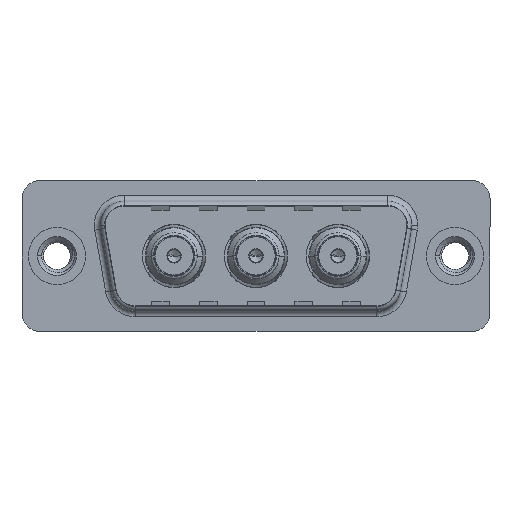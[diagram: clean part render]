
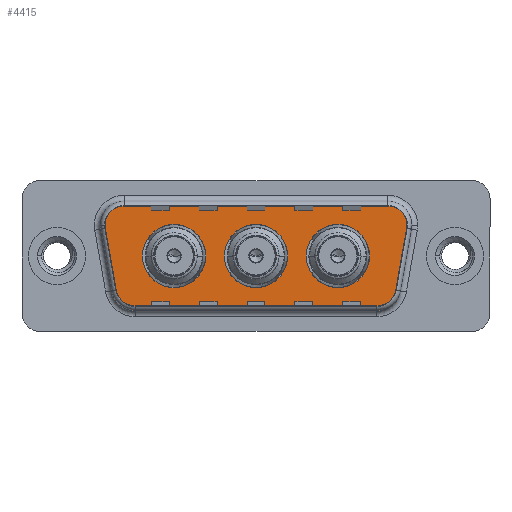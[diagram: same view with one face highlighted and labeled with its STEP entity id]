
A CAD part, top view. The second image highlights one B-rep face of the part: STEP entity #4415.
In plain terms, the highlighted planar face has unit normal (0, 0, 1).
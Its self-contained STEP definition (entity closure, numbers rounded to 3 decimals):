
#24 = ORIENTED_EDGE ( 'NONE', *, *, #8987, .F. ) ;
#173 = DIRECTION ( 'NONE',  ( 0., 0., 1. ) ) ;
#301 = DIRECTION ( 'NONE',  ( 0., 0., 1. ) ) ;
#363 = CIRCLE ( 'NONE', #13225, 2.65 ) ;
#427 = CARTESIAN_POINT ( 'NONE',  ( 16.65, 0., 0. ) ) ;
#432 = ORIENTED_EDGE ( 'NONE', *, *, #10453, .F. ) ;
#610 = AXIS2_PLACEMENT_3D ( 'NONE', #3767, #6325, #14634 ) ;
#1162 = DIRECTION ( 'NONE',  ( 0., 0., 1. ) ) ;
#1231 = AXIS2_PLACEMENT_3D ( 'NONE', #14390, #301, #10093 ) ;
#1262 = VERTEX_POINT ( 'NONE', #11161 ) ;
#1274 = CARTESIAN_POINT ( 'NONE',  ( 16.65, 0., 0. ) ) ;
#1303 = CARTESIAN_POINT ( 'NONE',  ( 7.15, 0., 0. ) ) ;
#1335 = DIRECTION ( 'NONE',  ( 0., 0., 1. ) ) ;
#1395 = CIRCLE ( 'NONE', #10770, 2.65 ) ;
#1501 = VECTOR ( 'NONE', #5473, 1000. ) ;
#1601 = CIRCLE ( 'NONE', #610, 2. ) ;
#1887 = AXIS2_PLACEMENT_3D ( 'NONE', #13021, #1162, #8384 ) ;
#1901 = CARTESIAN_POINT ( 'NONE',  ( 23.5, 0., 0. ) ) ;
#1971 = VERTEX_POINT ( 'NONE', #10240 ) ;
#1978 = ORIENTED_EDGE ( 'NONE', *, *, #2971, .F. ) ;
#2191 = CARTESIAN_POINT ( 'NONE',  ( 27.889, 2.9, 0. ) ) ;
#2239 = LINE ( 'NONE', #8644, #8415 ) ;
#2399 = FACE_BOUND ( 'NONE', #2434, .T. ) ;
#2434 = EDGE_LOOP ( 'NONE', ( #14392, #24 ) ) ;
#2557 = VERTEX_POINT ( 'NONE', #5701 ) ;
#2687 = EDGE_LOOP ( 'NONE', ( #15388, #13432, #11406, #6862, #10670, #14062, #4432, #4471, #3535 ) ) ;
#2800 = DIRECTION ( 'NONE',  ( 0., 0., 1. ) ) ;
#2971 = EDGE_CURVE ( 'NONE', #1262, #7063, #11347, .T. ) ;
#2984 = VERTEX_POINT ( 'NONE', #13394 ) ;
#3138 = DIRECTION ( 'NONE',  ( 1., 0., 0. ) ) ;
#3183 = CIRCLE ( 'NONE', #15477, 2. ) ;
#3528 = VECTOR ( 'NONE', #8202, 1000. ) ;
#3535 = ORIENTED_EDGE ( 'NONE', *, *, #8207, .T. ) ;
#3587 = CIRCLE ( 'NONE', #4645, 2.65 ) ;
#3723 = DIRECTION ( 'NONE',  ( 0.174, 0.985, 0. ) ) ;
#3767 = CARTESIAN_POINT ( 'NONE',  ( 5.411, 2.9, 0. ) ) ;
#3775 = CIRCLE ( 'NONE', #5178, 2.65 ) ;
#3802 = EDGE_CURVE ( 'NONE', #4691, #5275, #3183, .T. ) ;
#3902 = DIRECTION ( 'NONE',  ( 0., 0., 1. ) ) ;
#3920 = LINE ( 'NONE', #4544, #3528 ) ;
#3922 = DIRECTION ( 'NONE',  ( -1., 0., 0. ) ) ;
#4023 = EDGE_CURVE ( 'NONE', #7063, #1262, #3775, .T. ) ;
#4084 = DIRECTION ( 'NONE',  ( 0., 0., 1. ) ) ;
#4095 = CARTESIAN_POINT ( 'NONE',  ( 4.464, -3.247, 0. ) ) ;
#4415 = ADVANCED_FACE ( 'NONE', ( #9761, #2399, #8978, #15226 ), #9802, .T. ) ;
#4432 = ORIENTED_EDGE ( 'NONE', *, *, #12705, .T. ) ;
#4471 = ORIENTED_EDGE ( 'NONE', *, *, #3802, .T. ) ;
#4544 = CARTESIAN_POINT ( 'NONE',  ( 3.441, 2.553, 0. ) ) ;
#4645 = AXIS2_PLACEMENT_3D ( 'NONE', #7581, #173, #8822 ) ;
#4663 = CIRCLE ( 'NONE', #10992, 2. ) ;
#4691 = VERTEX_POINT ( 'NONE', #4095 ) ;
#4983 = ORIENTED_EDGE ( 'NONE', *, *, #4023, .F. ) ;
#5052 = EDGE_CURVE ( 'NONE', #7596, #10619, #1601, .T. ) ;
#5121 = DIRECTION ( 'NONE',  ( -1., 0., 0. ) ) ;
#5178 = AXIS2_PLACEMENT_3D ( 'NONE', #427, #3902, #14155 ) ;
#5256 = AXIS2_PLACEMENT_3D ( 'NONE', #1274, #1335, #8694 ) ;
#5275 = VERTEX_POINT ( 'NONE', #15960 ) ;
#5347 = CIRCLE ( 'NONE', #5966, 2.65 ) ;
#5382 = CARTESIAN_POINT ( 'NONE',  ( 26.866, -4.9, 0. ) ) ;
#5473 = DIRECTION ( 'NONE',  ( 1., 0., 0. ) ) ;
#5569 = EDGE_CURVE ( 'NONE', #12349, #10725, #14013, .T. ) ;
#5701 = CARTESIAN_POINT ( 'NONE',  ( 26.15, 0., 0. ) ) ;
#5815 = EDGE_LOOP ( 'NONE', ( #11433, #432 ) ) ;
#5966 = AXIS2_PLACEMENT_3D ( 'NONE', #14426, #6970, #15674 ) ;
#6082 = EDGE_CURVE ( 'NONE', #9436, #7174, #14394, .T. ) ;
#6321 = CARTESIAN_POINT ( 'NONE',  ( 29.889, 2.9, 0. ) ) ;
#6325 = DIRECTION ( 'NONE',  ( 0., 0., 1. ) ) ;
#6709 = VECTOR ( 'NONE', #15833, 1000. ) ;
#6862 = ORIENTED_EDGE ( 'NONE', *, *, #5569, .T. ) ;
#6970 = DIRECTION ( 'NONE',  ( 0., 0., 1. ) ) ;
#7063 = VERTEX_POINT ( 'NONE', #15761 ) ;
#7174 = VERTEX_POINT ( 'NONE', #7550 ) ;
#7308 = LINE ( 'NONE', #12887, #1501 ) ;
#7310 = CARTESIAN_POINT ( 'NONE',  ( 6.434, -2.9, 0. ) ) ;
#7550 = CARTESIAN_POINT ( 'NONE',  ( 28.836, -3.247, 0. ) ) ;
#7581 = CARTESIAN_POINT ( 'NONE',  ( 9.8, 0., 0. ) ) ;
#7596 = VERTEX_POINT ( 'NONE', #11562 ) ;
#7875 = DIRECTION ( 'NONE',  ( 0., 0., 1. ) ) ;
#8202 = DIRECTION ( 'NONE',  ( 0.174, -0.985, 0. ) ) ;
#8207 = EDGE_CURVE ( 'NONE', #5275, #9436, #7308, .T. ) ;
#8384 = DIRECTION ( 'NONE',  ( 1., 0., 0. ) ) ;
#8415 = VECTOR ( 'NONE', #3723, 1000. ) ;
#8501 = DIRECTION ( 'NONE',  ( 0., 0., 1. ) ) ;
#8613 = VERTEX_POINT ( 'NONE', #1303 ) ;
#8644 = CARTESIAN_POINT ( 'NONE',  ( 29.859, 2.553, 0. ) ) ;
#8694 = DIRECTION ( 'NONE',  ( 1., 0., 0. ) ) ;
#8822 = DIRECTION ( 'NONE',  ( 1., 0., 0. ) ) ;
#8978 = FACE_BOUND ( 'NONE', #5815, .T. ) ;
#8987 = EDGE_CURVE ( 'NONE', #1971, #2557, #5347, .T. ) ;
#9062 = CARTESIAN_POINT ( 'NONE',  ( 3.441, 2.553, 0. ) ) ;
#9085 = EDGE_CURVE ( 'NONE', #10725, #7596, #13719, .T. ) ;
#9196 = EDGE_CURVE ( 'NONE', #7174, #11336, #2239, .T. ) ;
#9436 = VERTEX_POINT ( 'NONE', #5382 ) ;
#9761 = FACE_BOUND ( 'NONE', #15566, .T. ) ;
#9802 = PLANE ( 'NONE',  #1231 ) ;
#10093 = DIRECTION ( 'NONE',  ( 1., 0., 0. ) ) ;
#10223 = CARTESIAN_POINT ( 'NONE',  ( 27.889, 2.9, 0. ) ) ;
#10240 = CARTESIAN_POINT ( 'NONE',  ( 20.85, 0., 0. ) ) ;
#10453 = EDGE_CURVE ( 'NONE', #8613, #2984, #3587, .T. ) ;
#10554 = DIRECTION ( 'NONE',  ( 0., 0., 1. ) ) ;
#10619 = VERTEX_POINT ( 'NONE', #9062 ) ;
#10670 = ORIENTED_EDGE ( 'NONE', *, *, #9085, .T. ) ;
#10725 = VERTEX_POINT ( 'NONE', #13256 ) ;
#10738 = CARTESIAN_POINT ( 'NONE',  ( 29.859, 2.553, 0. ) ) ;
#10770 = AXIS2_PLACEMENT_3D ( 'NONE', #1901, #10554, #3138 ) ;
#10992 = AXIS2_PLACEMENT_3D ( 'NONE', #10223, #2800, #11448 ) ;
#11161 = CARTESIAN_POINT ( 'NONE',  ( 14., 0., 0. ) ) ;
#11336 = VERTEX_POINT ( 'NONE', #10738 ) ;
#11347 = CIRCLE ( 'NONE', #5256, 2.65 ) ;
#11406 = ORIENTED_EDGE ( 'NONE', *, *, #13056, .T. ) ;
#11433 = ORIENTED_EDGE ( 'NONE', *, *, #15246, .F. ) ;
#11448 = DIRECTION ( 'NONE',  ( -1., 0., 0. ) ) ;
#11494 = CARTESIAN_POINT ( 'NONE',  ( 9.8, 0., 0. ) ) ;
#11562 = CARTESIAN_POINT ( 'NONE',  ( 5.411, 4.9, 0. ) ) ;
#12349 = VERTEX_POINT ( 'NONE', #6321 ) ;
#12616 = EDGE_CURVE ( 'NONE', #2557, #1971, #1395, .T. ) ;
#12705 = EDGE_CURVE ( 'NONE', #10619, #4691, #3920, .T. ) ;
#12754 = DIRECTION ( 'NONE',  ( 1., 0., 0. ) ) ;
#12887 = CARTESIAN_POINT ( 'NONE',  ( 6.434, -4.9, 0. ) ) ;
#13021 = CARTESIAN_POINT ( 'NONE',  ( 26.866, -2.9, 0. ) ) ;
#13056 = EDGE_CURVE ( 'NONE', #11336, #12349, #4663, .T. ) ;
#13225 = AXIS2_PLACEMENT_3D ( 'NONE', #11494, #4084, #12754 ) ;
#13256 = CARTESIAN_POINT ( 'NONE',  ( 27.889, 4.9, 0. ) ) ;
#13394 = CARTESIAN_POINT ( 'NONE',  ( 12.45, 0., 0. ) ) ;
#13432 = ORIENTED_EDGE ( 'NONE', *, *, #9196, .T. ) ;
#13719 = LINE ( 'NONE', #14584, #6709 ) ;
#14013 = CIRCLE ( 'NONE', #14455, 2. ) ;
#14062 = ORIENTED_EDGE ( 'NONE', *, *, #5052, .T. ) ;
#14155 = DIRECTION ( 'NONE',  ( 1., 0., 0. ) ) ;
#14390 = CARTESIAN_POINT ( 'NONE',  ( 26.866, -2.9, 0. ) ) ;
#14392 = ORIENTED_EDGE ( 'NONE', *, *, #12616, .F. ) ;
#14394 = CIRCLE ( 'NONE', #1887, 2. ) ;
#14426 = CARTESIAN_POINT ( 'NONE',  ( 23.5, 0., 0. ) ) ;
#14455 = AXIS2_PLACEMENT_3D ( 'NONE', #2191, #8501, #5121 ) ;
#14584 = CARTESIAN_POINT ( 'NONE',  ( 5.411, 4.9, 0. ) ) ;
#14634 = DIRECTION ( 'NONE',  ( 1., 0., 0. ) ) ;
#15226 = FACE_OUTER_BOUND ( 'NONE', #2687, .T. ) ;
#15246 = EDGE_CURVE ( 'NONE', #2984, #8613, #363, .T. ) ;
#15388 = ORIENTED_EDGE ( 'NONE', *, *, #6082, .T. ) ;
#15477 = AXIS2_PLACEMENT_3D ( 'NONE', #7310, #7875, #3922 ) ;
#15566 = EDGE_LOOP ( 'NONE', ( #4983, #1978 ) ) ;
#15674 = DIRECTION ( 'NONE',  ( 1., 0., 0. ) ) ;
#15761 = CARTESIAN_POINT ( 'NONE',  ( 19.3, 0., 0. ) ) ;
#15833 = DIRECTION ( 'NONE',  ( -1., 0., 0. ) ) ;
#15960 = CARTESIAN_POINT ( 'NONE',  ( 6.434, -4.9, 0. ) ) ;
